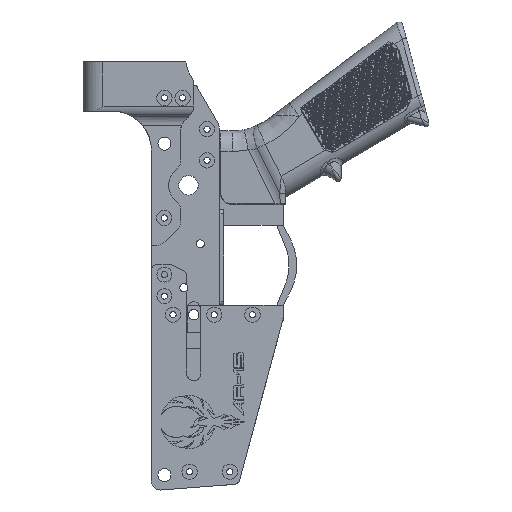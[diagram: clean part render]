
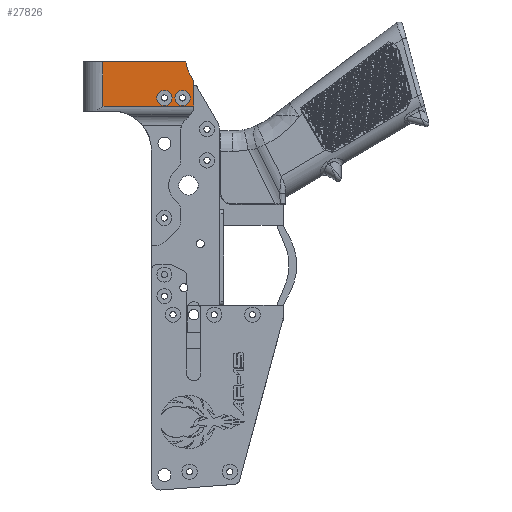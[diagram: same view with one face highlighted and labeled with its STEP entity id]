
A CAD part, left-side view. The second image highlights one B-rep face of the part: STEP entity #27826.
In plain terms, the highlighted planar face has unit normal (-1, 0, 0).
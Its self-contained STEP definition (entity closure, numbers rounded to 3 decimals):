
#469 = EDGE_CURVE ( 'NONE', #108803, #247844, #44404, .T. ) ;
#12295 = ORIENTED_EDGE ( 'NONE', *, *, #65253, .T. ) ;
#13675 = AXIS2_PLACEMENT_3D ( 'NONE', #114986, #177975, #133872 ) ;
#17334 = AXIS2_PLACEMENT_3D ( 'NONE', #126313, #109886, #203340 ) ;
#23381 = CARTESIAN_POINT ( 'NONE',  ( -25., 7.678, -10.291 ) ) ;
#25493 = VERTEX_POINT ( 'NONE', #23381 ) ;
#26951 = CARTESIAN_POINT ( 'NONE',  ( -25., -22.327, -6.35 ) ) ;
#27826 = ADVANCED_FACE ( 'NONE', ( #31507, #186883, #207090 ), #127574, .F. ) ;
#29424 = VECTOR ( 'NONE', #206711, 1000. ) ;
#31507 = FACE_BOUND ( 'NONE', #78588, .T. ) ;
#33145 = ORIENTED_EDGE ( 'NONE', *, *, #193549, .T. ) ;
#44404 = LINE ( 'NONE', #220001, #208008 ) ;
#45442 = EDGE_CURVE ( 'NONE', #78463, #104657, #85765, .T. ) ;
#49288 = ORIENTED_EDGE ( 'NONE', *, *, #156335, .T. ) ;
#49734 = ORIENTED_EDGE ( 'NONE', *, *, #195577, .F. ) ;
#49915 = AXIS2_PLACEMENT_3D ( 'NONE', #26951, #201276, #240433 ) ;
#50479 = CARTESIAN_POINT ( 'NONE',  ( -25., -36.779, -288600.29 ) ) ;
#53969 = EDGE_CURVE ( 'NONE', #130782, #179281, #68439, .T. ) ;
#54739 = CARTESIAN_POINT ( 'NONE',  ( -25., -36.779, -10.291 ) ) ;
#54800 = AXIS2_PLACEMENT_3D ( 'NONE', #50479, #130059, #204587 ) ;
#57414 = ORIENTED_EDGE ( 'NONE', *, *, #78496, .T. ) ;
#57992 = EDGE_CURVE ( 'NONE', #165074, #108803, #71849, .T. ) ;
#58449 = DIRECTION ( 'NONE',  ( 0., -1., 0. ) ) ;
#59363 = CARTESIAN_POINT ( 'NONE',  ( -25., 7.678, -12.776 ) ) ;
#60733 = EDGE_LOOP ( 'NONE', ( #49288, #57414, #229970, #193313, #12295, #33145 ) ) ;
#64038 = CARTESIAN_POINT ( 'NONE',  ( -25., -36.779, 1.76 ) ) ;
#65253 = EDGE_CURVE ( 'NONE', #247844, #222336, #101966, .T. ) ;
#67791 = DIRECTION ( 'NONE',  ( 0., 0., 1. ) ) ;
#68439 = CIRCLE ( 'NONE', #193392, 3.75 ) ;
#70729 = CARTESIAN_POINT ( 'NONE',  ( -25., -22.327, -2.6 ) ) ;
#71849 = LINE ( 'NONE', #129960, #238679 ) ;
#74377 = CARTESIAN_POINT ( 'NONE',  ( -25., -36.779, -10.291 ) ) ;
#75010 = CARTESIAN_POINT ( 'NONE',  ( -25., -32.853, 11.224 ) ) ;
#78463 = VERTEX_POINT ( 'NONE', #231527 ) ;
#78496 = EDGE_CURVE ( 'NONE', #25493, #165074, #134284, .T. ) ;
#78588 = EDGE_LOOP ( 'NONE', ( #182447, #49734 ) ) ;
#85765 = CIRCLE ( 'NONE', #113933, 3.75 ) ;
#89690 = CARTESIAN_POINT ( 'NONE',  ( -25., -22.327, -6.35 ) ) ;
#97512 = CARTESIAN_POINT ( 'NONE',  ( -25., -22.327, -10.1 ) ) ;
#101966 = CIRCLE ( 'NONE', #13675, 15. ) ;
#103854 = DIRECTION ( 'NONE',  ( 0., 0.5, 0.866 ) ) ;
#104657 = VERTEX_POINT ( 'NONE', #199421 ) ;
#108803 = VERTEX_POINT ( 'NONE', #64038 ) ;
#109886 = DIRECTION ( 'NONE',  ( -1., 0., 0. ) ) ;
#113933 = AXIS2_PLACEMENT_3D ( 'NONE', #141169, #240862, #67791 ) ;
#114201 = LINE ( 'NONE', #191190, #29424 ) ;
#114557 = VECTOR ( 'NONE', #58449, 1000. ) ;
#114986 = CARTESIAN_POINT ( 'NONE',  ( -25., -47.779, 12.707 ) ) ;
#119532 = ORIENTED_EDGE ( 'NONE', *, *, #130594, .F. ) ;
#126276 = CIRCLE ( 'NONE', #17334, 3.75 ) ;
#126313 = CARTESIAN_POINT ( 'NONE',  ( -25., -31.217, -6.35 ) ) ;
#127574 = PLANE ( 'NONE',  #54800 ) ;
#129960 = CARTESIAN_POINT ( 'NONE',  ( -25., -36.779, -288600.29 ) ) ;
#130059 = DIRECTION ( 'NONE',  ( 1., 0., 0. ) ) ;
#130594 = EDGE_CURVE ( 'NONE', #179281, #130782, #239673, .T. ) ;
#130782 = VERTEX_POINT ( 'NONE', #97512 ) ;
#132749 = CARTESIAN_POINT ( 'NONE',  ( -25., -34.789, 5.207 ) ) ;
#132877 = VECTOR ( 'NONE', #171870, 1000. ) ;
#133872 = DIRECTION ( 'NONE',  ( 0., 0., -1. ) ) ;
#134284 = LINE ( 'NONE', #54739, #114557 ) ;
#141169 = CARTESIAN_POINT ( 'NONE',  ( -25., -31.217, -6.35 ) ) ;
#156335 = EDGE_CURVE ( 'NONE', #165274, #25493, #232444, .T. ) ;
#165074 = VERTEX_POINT ( 'NONE', #74377 ) ;
#165274 = VERTEX_POINT ( 'NONE', #199290 ) ;
#166764 = DIRECTION ( 'NONE',  ( -1., 0., 0. ) ) ;
#171870 = DIRECTION ( 'NONE',  ( 0., 0., -1. ) ) ;
#175329 = EDGE_LOOP ( 'NONE', ( #119532, #236138 ) ) ;
#177975 = DIRECTION ( 'NONE',  ( 1., 0., 0. ) ) ;
#179281 = VERTEX_POINT ( 'NONE', #70729 ) ;
#182447 = ORIENTED_EDGE ( 'NONE', *, *, #45442, .F. ) ;
#184301 = DIRECTION ( 'NONE',  ( 0., 0., 1. ) ) ;
#186883 = FACE_BOUND ( 'NONE', #175329, .T. ) ;
#191190 = CARTESIAN_POINT ( 'NONE',  ( -25., -36.779, 11.224 ) ) ;
#193313 = ORIENTED_EDGE ( 'NONE', *, *, #469, .T. ) ;
#193392 = AXIS2_PLACEMENT_3D ( 'NONE', #89690, #166764, #243812 ) ;
#193549 = EDGE_CURVE ( 'NONE', #222336, #165274, #114201, .T. ) ;
#195577 = EDGE_CURVE ( 'NONE', #104657, #78463, #126276, .T. ) ;
#199290 = CARTESIAN_POINT ( 'NONE',  ( -25., 7.678, 11.224 ) ) ;
#199421 = CARTESIAN_POINT ( 'NONE',  ( -25., -31.217, -10.1 ) ) ;
#201276 = DIRECTION ( 'NONE',  ( -1., 0., 0. ) ) ;
#203340 = DIRECTION ( 'NONE',  ( 0., 0., 1. ) ) ;
#204587 = DIRECTION ( 'NONE',  ( 0., 0., -1. ) ) ;
#206711 = DIRECTION ( 'NONE',  ( 0., 1., 0. ) ) ;
#207090 = FACE_OUTER_BOUND ( 'NONE', #60733, .T. ) ;
#208008 = VECTOR ( 'NONE', #103854, 1000. ) ;
#220001 = CARTESIAN_POINT ( 'NONE',  ( -25., -32.779, 8.688 ) ) ;
#222336 = VERTEX_POINT ( 'NONE', #75010 ) ;
#229970 = ORIENTED_EDGE ( 'NONE', *, *, #57992, .T. ) ;
#231527 = CARTESIAN_POINT ( 'NONE',  ( -25., -31.217, -2.6 ) ) ;
#232444 = LINE ( 'NONE', #59363, #132877 ) ;
#236138 = ORIENTED_EDGE ( 'NONE', *, *, #53969, .F. ) ;
#238679 = VECTOR ( 'NONE', #184301, 1000. ) ;
#239673 = CIRCLE ( 'NONE', #49915, 3.75 ) ;
#240433 = DIRECTION ( 'NONE',  ( 0., 0., 1. ) ) ;
#240862 = DIRECTION ( 'NONE',  ( -1., 0., 0. ) ) ;
#243812 = DIRECTION ( 'NONE',  ( 0., 0., 1. ) ) ;
#247844 = VERTEX_POINT ( 'NONE', #132749 ) ;
